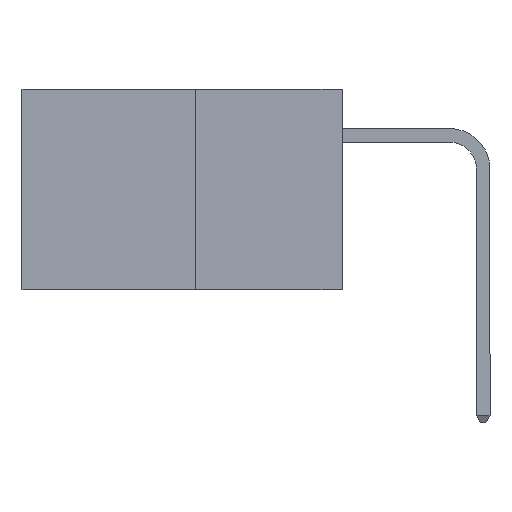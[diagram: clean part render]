
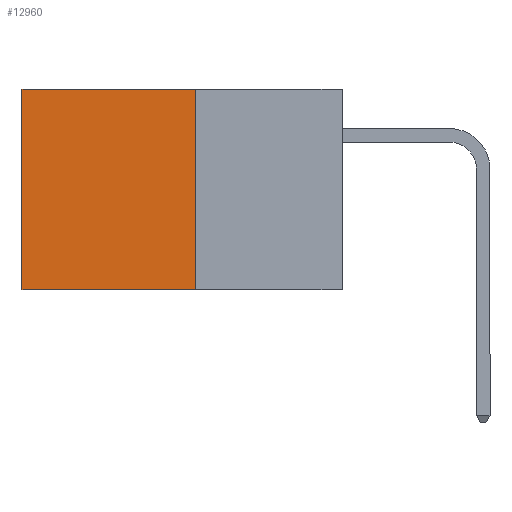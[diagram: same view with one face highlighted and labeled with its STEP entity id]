
A CAD part, left-side view. The second image highlights one B-rep face of the part: STEP entity #12960.
In plain terms, the highlighted planar face has unit normal (-1, 0, 0).
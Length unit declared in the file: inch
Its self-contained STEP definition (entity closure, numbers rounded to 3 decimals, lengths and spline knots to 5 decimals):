
#44 = CARTESIAN_POINT ( 'NONE',  ( 0.277, 0.59, -0.37 ) ) ;
#1541 = ORIENTED_EDGE ( 'NONE', *, *, #20657, .F. ) ;
#1604 = VERTEX_POINT ( 'NONE', #8420 ) ;
#2121 = CARTESIAN_POINT ( 'NONE',  ( 0.277, 0.27, -0.37 ) ) ;
#2378 = EDGE_CURVE ( 'NONE', #15850, #6633, #23763, .T. ) ;
#2524 = CARTESIAN_POINT ( 'NONE',  ( 0.277, 0.59, 0. ) ) ;
#3073 = ORIENTED_EDGE ( 'NONE', *, *, #5730, .T. ) ;
#3405 = VECTOR ( 'NONE', #18970, 39.37008 ) ;
#4164 = DIRECTION ( 'NONE',  ( 0., 0., -1. ) ) ;
#4763 = ORIENTED_EDGE ( 'NONE', *, *, #2378, .F. ) ;
#5730 = EDGE_CURVE ( 'NONE', #1604, #16662, #21455, .T. ) ;
#5824 = VECTOR ( 'NONE', #7206, 39.37008 ) ;
#6180 = PLANE ( 'NONE',  #16523 ) ;
#6633 = VERTEX_POINT ( 'NONE', #44 ) ;
#7206 = DIRECTION ( 'NONE',  ( 0., 1., 0. ) ) ;
#7289 = CARTESIAN_POINT ( 'NONE',  ( 0.277, 0.27, 0. ) ) ;
#8228 = EDGE_CURVE ( 'NONE', #16662, #6633, #20748, .T. ) ;
#8420 = CARTESIAN_POINT ( 'NONE',  ( 0.277, 0.27, 0. ) ) ;
#8481 = CARTESIAN_POINT ( 'NONE',  ( 0.277, 0.27, -0.37 ) ) ;
#9799 = DIRECTION ( 'NONE',  ( 0., 0., -1. ) ) ;
#10187 = CARTESIAN_POINT ( 'NONE',  ( 0.277, 0.27, -0.37 ) ) ;
#12109 = LINE ( 'NONE', #8481, #16895 ) ;
#12960 = ADVANCED_FACE ( 'NONE', ( #19047 ), #6180, .F. ) ;
#14069 = VECTOR ( 'NONE', #9799, 39.37008 ) ;
#14612 = EDGE_LOOP ( 'NONE', ( #23605, #4763, #1541, #3073 ) ) ;
#15850 = VERTEX_POINT ( 'NONE', #2121 ) ;
#16462 = DIRECTION ( 'NONE',  ( 1., 0., 0. ) ) ;
#16523 = AXIS2_PLACEMENT_3D ( 'NONE', #10187, #16462, #4164 ) ;
#16662 = VERTEX_POINT ( 'NONE', #2524 ) ;
#16669 = DIRECTION ( 'NONE',  ( 0., 0., -1. ) ) ;
#16895 = VECTOR ( 'NONE', #16669, 39.37008 ) ;
#18752 = CARTESIAN_POINT ( 'NONE',  ( 0.277, 0.27, -0.37 ) ) ;
#18970 = DIRECTION ( 'NONE',  ( 0., 1., 0. ) ) ;
#19047 = FACE_OUTER_BOUND ( 'NONE', #14612, .T. ) ;
#20657 = EDGE_CURVE ( 'NONE', #1604, #15850, #12109, .T. ) ;
#20748 = LINE ( 'NONE', #21932, #14069 ) ;
#21455 = LINE ( 'NONE', #7289, #5824 ) ;
#21932 = CARTESIAN_POINT ( 'NONE',  ( 0.277, 0.59, -0.37 ) ) ;
#23605 = ORIENTED_EDGE ( 'NONE', *, *, #8228, .T. ) ;
#23763 = LINE ( 'NONE', #18752, #3405 ) ;
